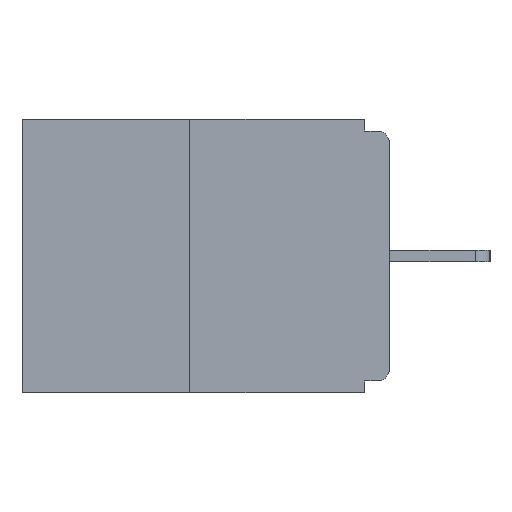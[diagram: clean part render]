
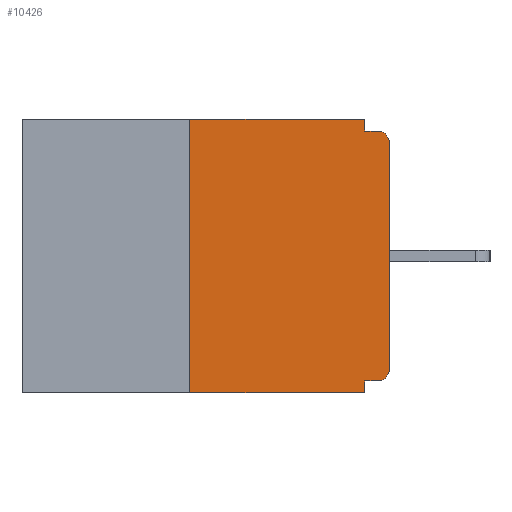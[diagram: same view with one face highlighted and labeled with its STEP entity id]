
A CAD part, left-side view. The second image highlights one B-rep face of the part: STEP entity #10426.
In plain terms, the highlighted planar face has unit normal (-1, 0, 0).
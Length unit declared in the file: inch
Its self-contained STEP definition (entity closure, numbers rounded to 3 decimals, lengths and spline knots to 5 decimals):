
#106 = CARTESIAN_POINT ( 'NONE',  ( 0., 0.031, -0.328 ) ) ;
#351 = DIRECTION ( 'NONE',  ( -1., 0., 0. ) ) ;
#530 = VERTEX_POINT ( 'NONE', #3549 ) ;
#902 = VERTEX_POINT ( 'NONE', #7251 ) ;
#1222 = CARTESIAN_POINT ( 'NONE',  ( 0., 0.031, 0. ) ) ;
#1684 = CARTESIAN_POINT ( 'NONE',  ( 0., 0.25, -0.343 ) ) ;
#1691 = VECTOR ( 'NONE', #7835, 39.37008 ) ;
#1716 = LINE ( 'NONE', #1222, #11505 ) ;
#2204 = EDGE_CURVE ( 'NONE', #9594, #3280, #4817, .T. ) ;
#2316 = ORIENTED_EDGE ( 'NONE', *, *, #6769, .F. ) ;
#2509 = VERTEX_POINT ( 'NONE', #1684 ) ;
#2762 = ORIENTED_EDGE ( 'NONE', *, *, #9690, .F. ) ;
#2834 = CARTESIAN_POINT ( 'NONE',  ( 0., 0.25, 0. ) ) ;
#3204 = VECTOR ( 'NONE', #4512, 39.37008 ) ;
#3210 = CIRCLE ( 'NONE', #15703, 0.015 ) ;
#3280 = VERTEX_POINT ( 'NONE', #12668 ) ;
#3549 = CARTESIAN_POINT ( 'NONE',  ( 0., 0.015, -0.015 ) ) ;
#3835 = CARTESIAN_POINT ( 'NONE',  ( 0., 0., -0.015 ) ) ;
#4028 = FACE_OUTER_BOUND ( 'NONE', #11093, .T. ) ;
#4124 = EDGE_CURVE ( 'NONE', #2509, #15868, #14133, .T. ) ;
#4150 = EDGE_CURVE ( 'NONE', #3280, #902, #11040, .T. ) ;
#4512 = DIRECTION ( 'NONE',  ( 0., 0., 1. ) ) ;
#4538 = VERTEX_POINT ( 'NONE', #7507 ) ;
#4817 = CIRCLE ( 'NONE', #9693, 0.015 ) ;
#5636 = DIRECTION ( 'NONE',  ( 0., 0., -1. ) ) ;
#6249 = AXIS2_PLACEMENT_3D ( 'NONE', #10628, #12964, #5636 ) ;
#6265 = CARTESIAN_POINT ( 'NONE',  ( 0., 0.46, 0. ) ) ;
#6288 = ORIENTED_EDGE ( 'NONE', *, *, #2204, .T. ) ;
#6541 = CARTESIAN_POINT ( 'NONE',  ( 0., 0.031, -0.343 ) ) ;
#6693 = ORIENTED_EDGE ( 'NONE', *, *, #7104, .F. ) ;
#6757 = CARTESIAN_POINT ( 'NONE',  ( 0., 0., -0.328 ) ) ;
#6769 = EDGE_CURVE ( 'NONE', #2509, #11366, #10016, .T. ) ;
#7104 = EDGE_CURVE ( 'NONE', #7295, #4538, #1716, .T. ) ;
#7251 = CARTESIAN_POINT ( 'NONE',  ( 0., 0., -0.03 ) ) ;
#7295 = VERTEX_POINT ( 'NONE', #13175 ) ;
#7410 = VECTOR ( 'NONE', #13363, 39.37008 ) ;
#7413 = DIRECTION ( 'NONE',  ( 0., -1., 0. ) ) ;
#7417 = CARTESIAN_POINT ( 'NONE',  ( 0., 0.46, -0.343 ) ) ;
#7484 = DIRECTION ( 'NONE',  ( -1., 0., 0. ) ) ;
#7507 = CARTESIAN_POINT ( 'NONE',  ( 0., 0.031, -0.015 ) ) ;
#7529 = LINE ( 'NONE', #6265, #13492 ) ;
#7573 = DIRECTION ( 'NONE',  ( 0., -1., 0. ) ) ;
#7835 = DIRECTION ( 'NONE',  ( 0., 0., -1. ) ) ;
#7912 = VECTOR ( 'NONE', #10194, 39.37008 ) ;
#8049 = DIRECTION ( 'NONE',  ( 0., 1., 0. ) ) ;
#8197 = CARTESIAN_POINT ( 'NONE',  ( 0., 0.031, -0.343 ) ) ;
#8277 = LINE ( 'NONE', #6541, #1691 ) ;
#8526 = VECTOR ( 'NONE', #8049, 39.37008 ) ;
#8633 = DIRECTION ( 'NONE',  ( 0., 0., -1. ) ) ;
#9594 = VERTEX_POINT ( 'NONE', #12585 ) ;
#9607 = ORIENTED_EDGE ( 'NONE', *, *, #4150, .T. ) ;
#9690 = EDGE_CURVE ( 'NONE', #9594, #10415, #15161, .T. ) ;
#9693 = AXIS2_PLACEMENT_3D ( 'NONE', #10402, #351, #8633 ) ;
#10016 = LINE ( 'NONE', #10812, #3204 ) ;
#10045 = EDGE_CURVE ( 'NONE', #902, #530, #3210, .T. ) ;
#10194 = DIRECTION ( 'NONE',  ( 0., -1., 0. ) ) ;
#10402 = CARTESIAN_POINT ( 'NONE',  ( 0., 0.015, -0.313 ) ) ;
#10415 = VERTEX_POINT ( 'NONE', #106 ) ;
#10426 = ADVANCED_FACE ( 'NONE', ( #4028 ), #10573, .F. ) ;
#10573 = PLANE ( 'NONE',  #6249 ) ;
#10628 = CARTESIAN_POINT ( 'NONE',  ( 0., 0.46, 0. ) ) ;
#10812 = CARTESIAN_POINT ( 'NONE',  ( 0., 0.25, 0. ) ) ;
#10813 = EDGE_CURVE ( 'NONE', #4538, #530, #14220, .T. ) ;
#11040 = LINE ( 'NONE', #11387, #7410 ) ;
#11093 = EDGE_LOOP ( 'NONE', ( #15121, #2316, #12378, #15485, #2762, #6288, #9607, #12749, #15852, #6693 ) ) ;
#11194 = EDGE_CURVE ( 'NONE', #10415, #15868, #8277, .T. ) ;
#11366 = VERTEX_POINT ( 'NONE', #2834 ) ;
#11387 = CARTESIAN_POINT ( 'NONE',  ( 0., 0., 0. ) ) ;
#11417 = VECTOR ( 'NONE', #7413, 39.37008 ) ;
#11505 = VECTOR ( 'NONE', #13737, 39.37008 ) ;
#12378 = ORIENTED_EDGE ( 'NONE', *, *, #4124, .T. ) ;
#12585 = CARTESIAN_POINT ( 'NONE',  ( 0., 0.015, -0.328 ) ) ;
#12668 = CARTESIAN_POINT ( 'NONE',  ( 0., 0., -0.313 ) ) ;
#12749 = ORIENTED_EDGE ( 'NONE', *, *, #10045, .T. ) ;
#12964 = DIRECTION ( 'NONE',  ( 1., 0., 0. ) ) ;
#13175 = CARTESIAN_POINT ( 'NONE',  ( 0., 0.031, 0. ) ) ;
#13363 = DIRECTION ( 'NONE',  ( 0., 0., 1. ) ) ;
#13492 = VECTOR ( 'NONE', #7573, 39.37008 ) ;
#13737 = DIRECTION ( 'NONE',  ( 0., 0., -1. ) ) ;
#14133 = LINE ( 'NONE', #7417, #11417 ) ;
#14220 = LINE ( 'NONE', #3835, #7912 ) ;
#14613 = CARTESIAN_POINT ( 'NONE',  ( 0., 0.015, -0.03 ) ) ;
#14961 = EDGE_CURVE ( 'NONE', #11366, #7295, #7529, .T. ) ;
#15121 = ORIENTED_EDGE ( 'NONE', *, *, #14961, .F. ) ;
#15161 = LINE ( 'NONE', #6757, #8526 ) ;
#15485 = ORIENTED_EDGE ( 'NONE', *, *, #11194, .F. ) ;
#15703 = AXIS2_PLACEMENT_3D ( 'NONE', #14613, #7484, #15780 ) ;
#15780 = DIRECTION ( 'NONE',  ( 0., 0., -1. ) ) ;
#15852 = ORIENTED_EDGE ( 'NONE', *, *, #10813, .F. ) ;
#15868 = VERTEX_POINT ( 'NONE', #8197 ) ;
